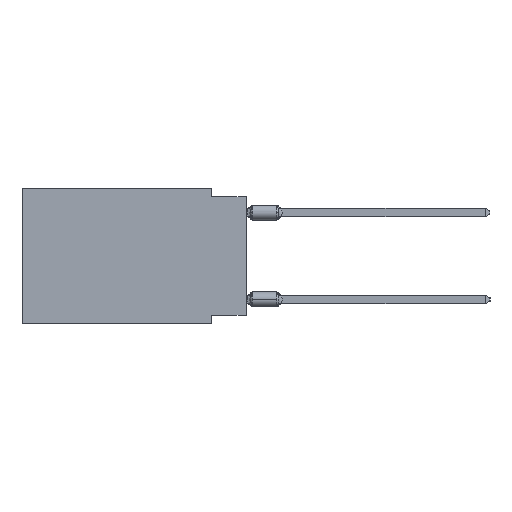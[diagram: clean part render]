
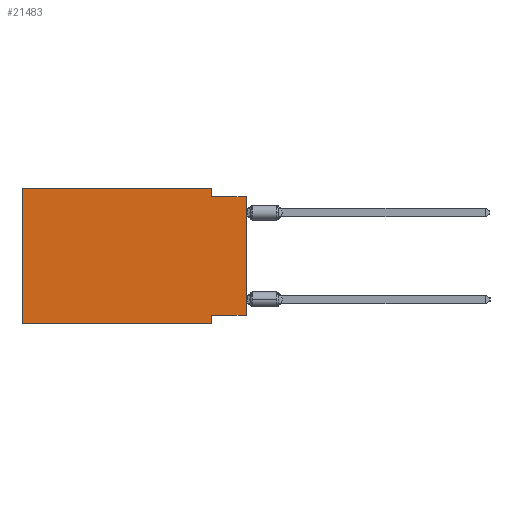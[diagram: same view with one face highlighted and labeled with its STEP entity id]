
A CAD part, left-side view. The second image highlights one B-rep face of the part: STEP entity #21483.
In plain terms, the highlighted planar face has unit normal (-1, 0, 0).
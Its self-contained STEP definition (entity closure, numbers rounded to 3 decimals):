
#509 = LINE ( 'NONE', #7319, #43491 ) ;
#517 = VECTOR ( 'NONE', #36572, 1000. ) ;
#941 = DIRECTION ( 'NONE',  ( 0., 0., 1. ) ) ;
#1576 = VECTOR ( 'NONE', #16493, 1000. ) ;
#1679 = CARTESIAN_POINT ( 'NONE',  ( 0., 16.383, -9.906 ) ) ;
#2741 = ORIENTED_EDGE ( 'NONE', *, *, #41590, .T. ) ;
#3301 = VERTEX_POINT ( 'NONE', #37155 ) ;
#3515 = LINE ( 'NONE', #21485, #26698 ) ;
#4152 = CARTESIAN_POINT ( 'NONE',  ( 0., 2.54, -9.271 ) ) ;
#4903 = EDGE_CURVE ( 'NONE', #13899, #21692, #24350, .T. ) ;
#7226 = ORIENTED_EDGE ( 'NONE', *, *, #16391, .F. ) ;
#7319 = CARTESIAN_POINT ( 'NONE',  ( 0., 0., -9.271 ) ) ;
#7389 = CARTESIAN_POINT ( 'NONE',  ( 0., 0., -0.635 ) ) ;
#7574 = EDGE_CURVE ( 'NONE', #39793, #34863, #509, .T. ) ;
#8121 = EDGE_CURVE ( 'NONE', #39793, #20953, #26904, .T. ) ;
#8181 = ORIENTED_EDGE ( 'NONE', *, *, #28710, .F. ) ;
#10267 = AXIS2_PLACEMENT_3D ( 'NONE', #21876, #17508, #36891 ) ;
#10358 = CARTESIAN_POINT ( 'NONE',  ( 0., 2.54, 0. ) ) ;
#11244 = EDGE_CURVE ( 'NONE', #13751, #20953, #43814, .T. ) ;
#11264 = EDGE_CURVE ( 'NONE', #34863, #3301, #3515, .T. ) ;
#11851 = CARTESIAN_POINT ( 'NONE',  ( 0., 0., -9.271 ) ) ;
#12363 = LINE ( 'NONE', #1679, #1576 ) ;
#13751 = VERTEX_POINT ( 'NONE', #47073 ) ;
#13899 = VERTEX_POINT ( 'NONE', #19555 ) ;
#14844 = DIRECTION ( 'NONE',  ( 0., 1., 0. ) ) ;
#15199 = ORIENTED_EDGE ( 'NONE', *, *, #4903, .F. ) ;
#16391 = EDGE_CURVE ( 'NONE', #34682, #13899, #40455, .T. ) ;
#16493 = DIRECTION ( 'NONE',  ( 0., -1., 0. ) ) ;
#17508 = DIRECTION ( 'NONE',  ( 1., 0., 0. ) ) ;
#19555 = CARTESIAN_POINT ( 'NONE',  ( 0., 16.383, 0. ) ) ;
#20271 = VECTOR ( 'NONE', #941, 1000. ) ;
#20953 = VERTEX_POINT ( 'NONE', #30758 ) ;
#21301 = CARTESIAN_POINT ( 'NONE',  ( 0., 16.383, 0. ) ) ;
#21483 = ADVANCED_FACE ( 'NONE', ( #36657 ), #24787, .F. ) ;
#21485 = CARTESIAN_POINT ( 'NONE',  ( 0., 2.54, -9.906 ) ) ;
#21692 = VERTEX_POINT ( 'NONE', #41980 ) ;
#21876 = CARTESIAN_POINT ( 'NONE',  ( 0., 16.383, 0. ) ) ;
#23050 = ORIENTED_EDGE ( 'NONE', *, *, #11244, .F. ) ;
#23266 = CARTESIAN_POINT ( 'NONE',  ( 0., 0., 0. ) ) ;
#24350 = LINE ( 'NONE', #35258, #36316 ) ;
#24441 = LINE ( 'NONE', #10358, #47941 ) ;
#24677 = DIRECTION ( 'NONE',  ( 0., 0., -1. ) ) ;
#24787 = PLANE ( 'NONE',  #10267 ) ;
#26105 = ORIENTED_EDGE ( 'NONE', *, *, #8121, .T. ) ;
#26315 = DIRECTION ( 'NONE',  ( 0., 0., -1. ) ) ;
#26698 = VECTOR ( 'NONE', #26315, 1000. ) ;
#26801 = ORIENTED_EDGE ( 'NONE', *, *, #7574, .F. ) ;
#26904 = LINE ( 'NONE', #23266, #20271 ) ;
#28710 = EDGE_CURVE ( 'NONE', #21692, #13751, #24441, .T. ) ;
#30758 = CARTESIAN_POINT ( 'NONE',  ( 0., 0., -0.635 ) ) ;
#33735 = ORIENTED_EDGE ( 'NONE', *, *, #11264, .F. ) ;
#34682 = VERTEX_POINT ( 'NONE', #35707 ) ;
#34863 = VERTEX_POINT ( 'NONE', #4152 ) ;
#35192 = VECTOR ( 'NONE', #40864, 1000. ) ;
#35258 = CARTESIAN_POINT ( 'NONE',  ( 0., 16.383, 0. ) ) ;
#35707 = CARTESIAN_POINT ( 'NONE',  ( 0., 16.383, -9.906 ) ) ;
#36316 = VECTOR ( 'NONE', #43033, 1000. ) ;
#36395 = EDGE_LOOP ( 'NONE', ( #26105, #23050, #8181, #15199, #7226, #2741, #33735, #26801 ) ) ;
#36572 = DIRECTION ( 'NONE',  ( 0., 0., 1. ) ) ;
#36657 = FACE_OUTER_BOUND ( 'NONE', #36395, .T. ) ;
#36891 = DIRECTION ( 'NONE',  ( 0., 0., -1. ) ) ;
#37155 = CARTESIAN_POINT ( 'NONE',  ( 0., 2.54, -9.906 ) ) ;
#39793 = VERTEX_POINT ( 'NONE', #11851 ) ;
#40455 = LINE ( 'NONE', #21301, #517 ) ;
#40864 = DIRECTION ( 'NONE',  ( 0., -1., 0. ) ) ;
#41590 = EDGE_CURVE ( 'NONE', #34682, #3301, #12363, .T. ) ;
#41980 = CARTESIAN_POINT ( 'NONE',  ( 0., 2.54, 0. ) ) ;
#43033 = DIRECTION ( 'NONE',  ( 0., -1., 0. ) ) ;
#43491 = VECTOR ( 'NONE', #14844, 1000. ) ;
#43814 = LINE ( 'NONE', #7389, #35192 ) ;
#47073 = CARTESIAN_POINT ( 'NONE',  ( 0., 2.54, -0.635 ) ) ;
#47941 = VECTOR ( 'NONE', #24677, 1000. ) ;
